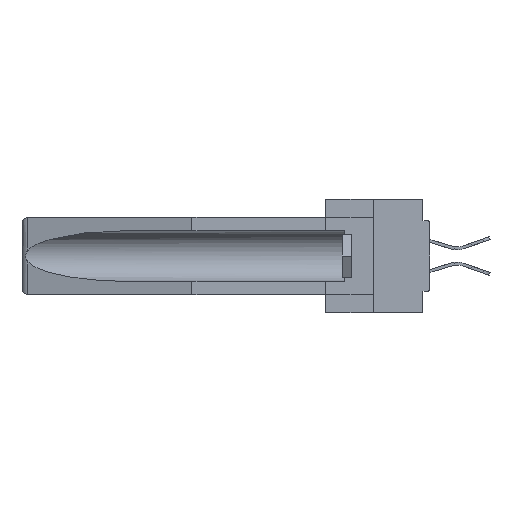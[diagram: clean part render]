
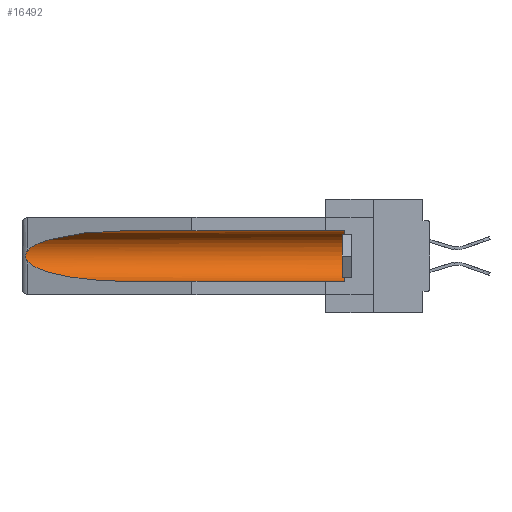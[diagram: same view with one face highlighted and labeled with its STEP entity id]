
A CAD part, left-side view. The second image highlights one B-rep face of the part: STEP entity #16492.
In plain terms, the highlighted cylindrical face has radius 2.857 mm (diameter 5.715 mm), a partial arc.
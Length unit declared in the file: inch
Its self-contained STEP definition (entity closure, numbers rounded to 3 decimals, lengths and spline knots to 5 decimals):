
#1663 = DIRECTION ( 'NONE',  ( 0., 0., 1. ) ) ;
#1790 = CARTESIAN_POINT ( 'NONE',  ( 0.155, -0.30754, -0.1715 ) ) ;
#2144 = CARTESIAN_POINT ( 'NONE',  ( 0.26537, 1.52718, -0.19328 ) ) ;
#2218 = CARTESIAN_POINT ( 'NONE',  ( 0.155, 1.07973, -0.284 ) ) ;
#4422 = CARTESIAN_POINT ( 'NONE',  ( 0.155, 0.126, -0.1715 ) ) ;
#5034 = ORIENTED_EDGE ( 'NONE', *, *, #37089, .T. ) ;
#5119 = VECTOR ( 'NONE', #25915, 39.37008 ) ;
#5491 = CARTESIAN_POINT ( 'NONE',  ( 0.26597, 1.5296, -0.19026 ) ) ;
#5705 = VECTOR ( 'NONE', #13410, 39.37008 ) ;
#5860 = CARTESIAN_POINT ( 'NONE',  ( 0.155, 0.126, -0.059 ) ) ;
#5889 =( BOUNDED_CURVE ( )  B_SPLINE_CURVE ( 3, ( #18982, #40779, #37625, #21891 ),
 .UNSPECIFIED., .F., .T. ) 
 B_SPLINE_CURVE_WITH_KNOTS ( ( 4, 4 ),
 ( 0.1948, 1.5708 ),
 .UNSPECIFIED. ) 
 CURVE ( )  GEOMETRIC_REPRESENTATION_ITEM ( )  RATIONAL_B_SPLINE_CURVE ( ( 1., 0.848, 0.848, 1. ) ) 
 REPRESENTATION_ITEM ( '' )  );
#8651 = CARTESIAN_POINT ( 'NONE',  ( 0.2675, 1.53308, -0.16763 ) ) ;
#9779 = VERTEX_POINT ( 'NONE', #36611 ) ;
#10523 = EDGE_CURVE ( 'NONE', #26258, #15551, #24826, .T. ) ;
#11217 = CARTESIAN_POINT ( 'NONE',  ( 0.26537, 1.52718, -0.19328 ) ) ;
#11709 = AXIS2_PLACEMENT_3D ( 'NONE', #4422, #32387, #19705 ) ;
#11796 = CARTESIAN_POINT ( 'NONE',  ( 0.2673, 1.53269, -0.17917 ) ) ;
#12086 = CARTESIAN_POINT ( 'NONE',  ( 0.26655, 1.53094, -0.18657 ) ) ;
#13410 = DIRECTION ( 'NONE',  ( 0., 1., 0. ) ) ;
#14730 = CARTESIAN_POINT ( 'NONE',  ( 0.2673, 1.5327, -0.16383 ) ) ;
#15551 = VERTEX_POINT ( 'NONE', #2218 ) ;
#15842 = EDGE_CURVE ( 'NONE', #26258, #29155, #40708, .T. ) ;
#16195 = CARTESIAN_POINT ( 'NONE',  ( 0.155, 0.126, -0.284 ) ) ;
#16492 = ADVANCED_FACE ( 'NONE', ( #20396 ), #30269, .F. ) ;
#16939 = VERTEX_POINT ( 'NONE', #11217 ) ;
#17145 = ORIENTED_EDGE ( 'NONE', *, *, #35525, .T. ) ;
#18273 = CARTESIAN_POINT ( 'NONE',  ( 0.26597, 1.52961, -0.15275 ) ) ;
#18982 = CARTESIAN_POINT ( 'NONE',  ( 0.26537, 1.52718, -0.19328 ) ) ;
#19495 = CARTESIAN_POINT ( 'NONE',  ( 0.26537, 1.52718, -0.14972 ) ) ;
#19705 = DIRECTION ( 'NONE',  ( 0., 0., 1. ) ) ;
#20396 = FACE_OUTER_BOUND ( 'NONE', #28445, .T. ) ;
#20720 = AXIS2_PLACEMENT_3D ( 'NONE', #1790, #26983, #1663 ) ;
#21305 = CARTESIAN_POINT ( 'NONE',  ( 0.26537, 1.52718, -0.14972 ) ) ;
#21891 = CARTESIAN_POINT ( 'NONE',  ( 0.155, 1.07973, -0.284 ) ) ;
#22400 = LINE ( 'NONE', #32120, #5705 ) ;
#22725 = ORIENTED_EDGE ( 'NONE', *, *, #30362, .T. ) ;
#22746 = CARTESIAN_POINT ( 'NONE',  ( 0.155, -0.30754, -0.284 ) ) ;
#24172 = CARTESIAN_POINT ( 'NONE',  ( 0.26654, 1.53092, -0.15636 ) ) ;
#24826 = LINE ( 'NONE', #22746, #5119 ) ;
#25915 = DIRECTION ( 'NONE',  ( 0., 1., 0. ) ) ;
#26258 = VERTEX_POINT ( 'NONE', #16195 ) ;
#26980 = ORIENTED_EDGE ( 'NONE', *, *, #10523, .F. ) ;
#26983 = DIRECTION ( 'NONE',  ( 0., 1., 0. ) ) ;
#27140 = VERTEX_POINT ( 'NONE', #37166 ) ;
#28445 = EDGE_LOOP ( 'NONE', ( #17145, #5034, #22725, #26980, #32668, #38437 ) ) ;
#28558 = B_SPLINE_CURVE_WITH_KNOTS ( 'NONE', 3,
 ( #21305, #18273, #24172, #14730, #8651, #40478, #11796, #12086, #5491, #2144 ),
 .UNSPECIFIED., .F., .F.,
 ( 4, 2, 2, 2, 4 ),
 ( 0., 0.00029, 0.00058, 0.00087, 0.00117 ),
 .UNSPECIFIED. ) ;
#29155 = VERTEX_POINT ( 'NONE', #5860 ) ;
#30269 = CYLINDRICAL_SURFACE ( 'NONE', #20720, 0.1125 ) ;
#30362 = EDGE_CURVE ( 'NONE', #16939, #15551, #5889, .T. ) ;
#31762 = CARTESIAN_POINT ( 'NONE',  ( 0.25451, 1.48313, -0.09465 ) ) ;
#32120 = CARTESIAN_POINT ( 'NONE',  ( 0.155, -0.30754, -0.059 ) ) ;
#32170 = CARTESIAN_POINT ( 'NONE',  ( 0.21114, 1.30732, -0.059 ) ) ;
#32387 = DIRECTION ( 'NONE',  ( 0., -1., 0. ) ) ;
#32668 = ORIENTED_EDGE ( 'NONE', *, *, #15842, .T. ) ;
#32868 =( BOUNDED_CURVE ( )  B_SPLINE_CURVE ( 3, ( #38400, #32170, #31762, #19495 ),
 .UNSPECIFIED., .F., .T. ) 
 B_SPLINE_CURVE_WITH_KNOTS ( ( 4, 4 ),
 ( 4.71239, 6.08839 ),
 .UNSPECIFIED. ) 
 CURVE ( )  GEOMETRIC_REPRESENTATION_ITEM ( )  RATIONAL_B_SPLINE_CURVE ( ( 1., 0.848, 0.848, 1. ) ) 
 REPRESENTATION_ITEM ( '' )  );
#35525 = EDGE_CURVE ( 'NONE', #27140, #9779, #32868, .T. ) ;
#36611 = CARTESIAN_POINT ( 'NONE',  ( 0.26537, 1.52718, -0.14972 ) ) ;
#37089 = EDGE_CURVE ( 'NONE', #9779, #16939, #28558, .T. ) ;
#37166 = CARTESIAN_POINT ( 'NONE',  ( 0.155, 1.07973, -0.059 ) ) ;
#37625 = CARTESIAN_POINT ( 'NONE',  ( 0.21114, 1.30732, -0.284 ) ) ;
#38400 = CARTESIAN_POINT ( 'NONE',  ( 0.155, 1.07973, -0.059 ) ) ;
#38437 = ORIENTED_EDGE ( 'NONE', *, *, #39276, .T. ) ;
#39276 = EDGE_CURVE ( 'NONE', #29155, #27140, #22400, .T. ) ;
#40478 = CARTESIAN_POINT ( 'NONE',  ( 0.2675, 1.53308, -0.17534 ) ) ;
#40708 = CIRCLE ( 'NONE', #11709, 0.1125 ) ;
#40779 = CARTESIAN_POINT ( 'NONE',  ( 0.25451, 1.48313, -0.24835 ) ) ;
